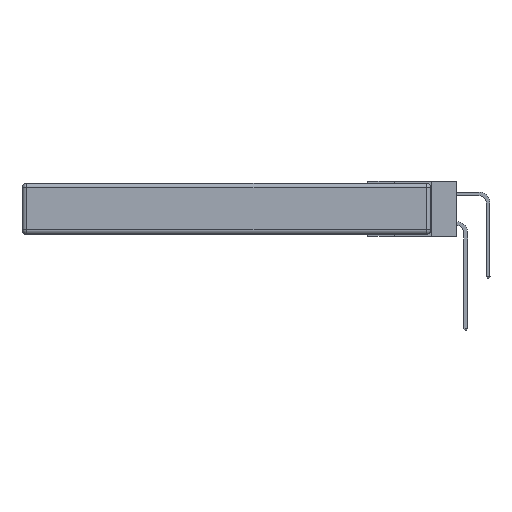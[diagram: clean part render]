
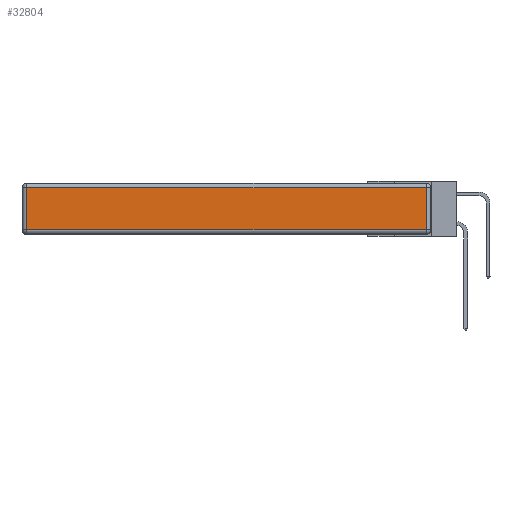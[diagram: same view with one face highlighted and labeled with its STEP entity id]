
A CAD part, left-side view. The second image highlights one B-rep face of the part: STEP entity #32804.
In plain terms, the highlighted planar face has unit normal (-1, 0, 0).
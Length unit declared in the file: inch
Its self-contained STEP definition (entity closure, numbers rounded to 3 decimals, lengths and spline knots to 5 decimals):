
#2656 = VECTOR ( 'NONE', #23104, 39.37008 ) ;
#5022 = EDGE_CURVE ( 'NONE', #30889, #24326, #26879, .T. ) ;
#6313 = ORIENTED_EDGE ( 'NONE', *, *, #20107, .T. ) ;
#7160 = CARTESIAN_POINT ( 'NONE',  ( 0., 0.03, -0.313 ) ) ;
#7352 = ORIENTED_EDGE ( 'NONE', *, *, #5022, .T. ) ;
#9003 = CARTESIAN_POINT ( 'NONE',  ( 0., 0., -0.343 ) ) ;
#11771 = PLANE ( 'NONE',  #25845 ) ;
#13393 = CARTESIAN_POINT ( 'NONE',  ( 0., 0.03, -0.03 ) ) ;
#13619 = DIRECTION ( 'NONE',  ( 0., 0., 1. ) ) ;
#15220 = EDGE_CURVE ( 'NONE', #19276, #30889, #33628, .T. ) ;
#16917 = CARTESIAN_POINT ( 'NONE',  ( 0., 2.72, -0.343 ) ) ;
#19199 = CARTESIAN_POINT ( 'NONE',  ( 0., 2.72, -0.313 ) ) ;
#19276 = VERTEX_POINT ( 'NONE', #7160 ) ;
#19442 = DIRECTION ( 'NONE',  ( 0., 0., -1. ) ) ;
#20107 = EDGE_CURVE ( 'NONE', #28735, #19276, #30151, .T. ) ;
#21174 = CARTESIAN_POINT ( 'NONE',  ( 0., 2.72, -0.03 ) ) ;
#21869 = CARTESIAN_POINT ( 'NONE',  ( 0., 0., -0.313 ) ) ;
#21882 = VECTOR ( 'NONE', #26832, 39.37008 ) ;
#22091 = VECTOR ( 'NONE', #13619, 39.37008 ) ;
#23104 = DIRECTION ( 'NONE',  ( 0., 1., 0. ) ) ;
#24326 = VERTEX_POINT ( 'NONE', #21174 ) ;
#24906 = FACE_OUTER_BOUND ( 'NONE', #29425, .T. ) ;
#25620 = ORIENTED_EDGE ( 'NONE', *, *, #33774, .T. ) ;
#25845 = AXIS2_PLACEMENT_3D ( 'NONE', #9003, #30111, #30361 ) ;
#26234 = CARTESIAN_POINT ( 'NONE',  ( 0., 0.03, -0.343 ) ) ;
#26832 = DIRECTION ( 'NONE',  ( 0., -1., 0. ) ) ;
#26879 = LINE ( 'NONE', #33207, #2656 ) ;
#27443 = ORIENTED_EDGE ( 'NONE', *, *, #15220, .T. ) ;
#28490 = LINE ( 'NONE', #16917, #32578 ) ;
#28735 = VERTEX_POINT ( 'NONE', #19199 ) ;
#29425 = EDGE_LOOP ( 'NONE', ( #6313, #27443, #7352, #25620 ) ) ;
#30111 = DIRECTION ( 'NONE',  ( -1., 0., 0. ) ) ;
#30151 = LINE ( 'NONE', #21869, #21882 ) ;
#30361 = DIRECTION ( 'NONE',  ( 0., 0., 1. ) ) ;
#30889 = VERTEX_POINT ( 'NONE', #13393 ) ;
#32578 = VECTOR ( 'NONE', #19442, 39.37008 ) ;
#32804 = ADVANCED_FACE ( 'NONE', ( #24906 ), #11771, .T. ) ;
#33207 = CARTESIAN_POINT ( 'NONE',  ( 0., 2.75, -0.03 ) ) ;
#33628 = LINE ( 'NONE', #26234, #22091 ) ;
#33774 = EDGE_CURVE ( 'NONE', #24326, #28735, #28490, .T. ) ;
